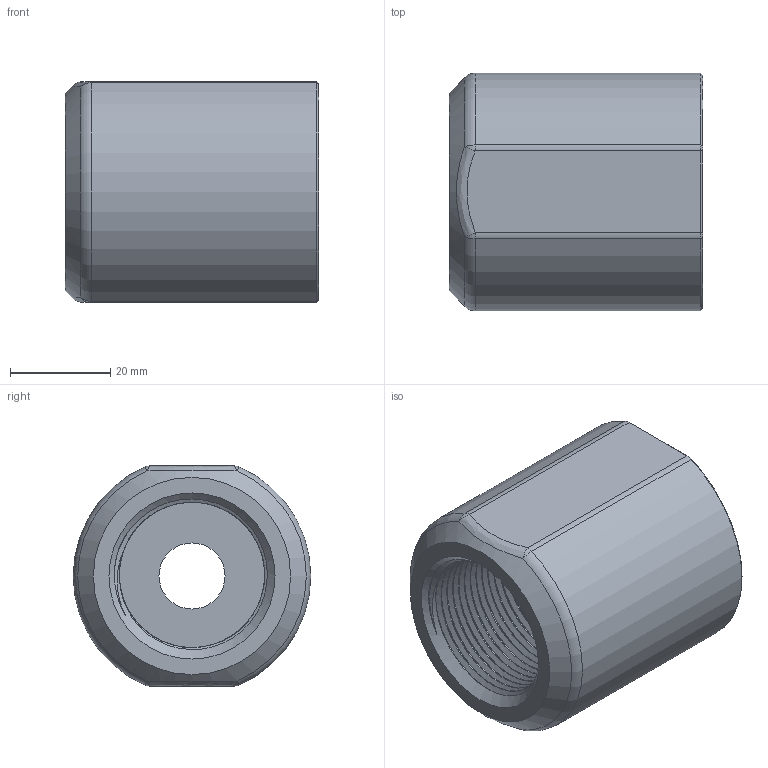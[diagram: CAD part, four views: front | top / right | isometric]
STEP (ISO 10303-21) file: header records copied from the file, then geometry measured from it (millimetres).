
FILE_DESCRIPTION (( 'STEP AP203' ), '1' );
FILE_NAME ('MOD9_threaded_stock_adapter.STEP', '2020-06-10T05:01:07', ( '' ), ( '' ), 'SwSTEP 2.0', 'SolidWorks 2016', '' );
FILE_SCHEMA (( 'CONFIG_CONTROL_DESIGN' ));
Length unit declared in the file: millimetre
Products named in the file (1): MOD9_threaded_stock_adapter
Bounding box: 50.61 x 47.42 x 44.06 mm (x, y, z)
Volume: 54911.8 mm3; surface area: 16570.2 mm2
Topology: 1 solids, 1 shells, 70 faces, 163 edges, 97 vertices
Faces by surface type: plane 24, cone 17, bspline 12, cylinder 11, sphere 4, torus 2
Full cylindrical faces by diameter (mm): 13.177 x1
Entity records: 9263 total; most frequent: CARTESIAN_POINT 7762, ORIENTED_EDGE 314, DIRECTION 268, EDGE_CURVE 157, AXIS2_PLACEMENT_3D 104, VERTEX_POINT 95, EDGE_LOOP 78, FACE_OUTER_BOUND 71
